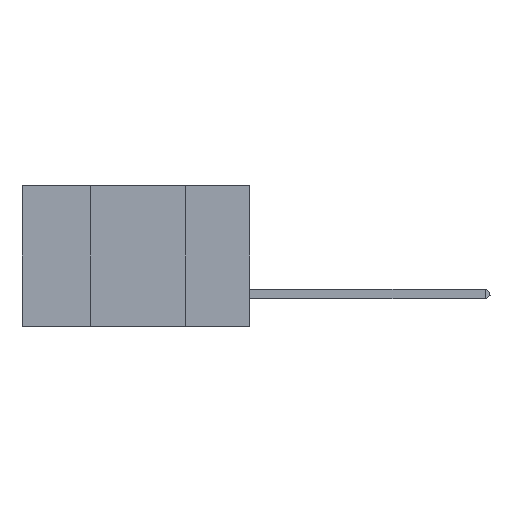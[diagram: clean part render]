
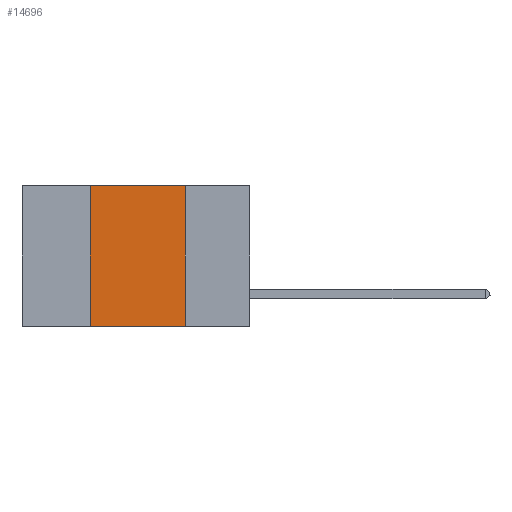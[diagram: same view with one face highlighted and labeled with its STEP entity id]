
A CAD part, left-side view. The second image highlights one B-rep face of the part: STEP entity #14696.
In plain terms, the highlighted planar face has unit normal (-1, 0, 0).
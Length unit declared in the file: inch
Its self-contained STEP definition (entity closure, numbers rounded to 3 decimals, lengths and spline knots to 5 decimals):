
#345 = LINE ( 'NONE', #9180, #18516 ) ;
#493 = VECTOR ( 'NONE', #5244, 39.37008 ) ;
#888 = VERTEX_POINT ( 'NONE', #1486 ) ;
#1486 = CARTESIAN_POINT ( 'NONE',  ( 0., 0.17, -0.37 ) ) ;
#1502 = CARTESIAN_POINT ( 'NONE',  ( 0., 0.6, -0.37 ) ) ;
#2614 = DIRECTION ( 'NONE',  ( 0., 0., 1. ) ) ;
#3941 = DIRECTION ( 'NONE',  ( 0., 0., -1. ) ) ;
#4021 = LINE ( 'NONE', #1502, #16399 ) ;
#4168 = DIRECTION ( 'NONE',  ( 1., 0., 0. ) ) ;
#4322 = VECTOR ( 'NONE', #19397, 39.37008 ) ;
#5244 = DIRECTION ( 'NONE',  ( 0., -1., 0. ) ) ;
#5332 = EDGE_CURVE ( 'NONE', #5375, #17509, #345, .T. ) ;
#5375 = VERTEX_POINT ( 'NONE', #17888 ) ;
#6744 = ORIENTED_EDGE ( 'NONE', *, *, #5332, .F. ) ;
#7427 = ORIENTED_EDGE ( 'NONE', *, *, #18509, .F. ) ;
#8189 = AXIS2_PLACEMENT_3D ( 'NONE', #19350, #4168, #3941 ) ;
#8877 = ORIENTED_EDGE ( 'NONE', *, *, #14952, .F. ) ;
#9180 = CARTESIAN_POINT ( 'NONE',  ( 0., 0.42, 0. ) ) ;
#10536 = LINE ( 'NONE', #15201, #493 ) ;
#12837 = EDGE_CURVE ( 'NONE', #5375, #888, #4021, .T. ) ;
#12891 = FACE_OUTER_BOUND ( 'NONE', #15866, .T. ) ;
#13281 = LINE ( 'NONE', #19268, #4322 ) ;
#14696 = ADVANCED_FACE ( 'NONE', ( #12891 ), #20930, .F. ) ;
#14952 = EDGE_CURVE ( 'NONE', #17509, #15002, #10536, .T. ) ;
#15002 = VERTEX_POINT ( 'NONE', #17249 ) ;
#15201 = CARTESIAN_POINT ( 'NONE',  ( 0., 0.6, 0. ) ) ;
#15866 = EDGE_LOOP ( 'NONE', ( #7427, #8877, #6744, #16803 ) ) ;
#16399 = VECTOR ( 'NONE', #19965, 39.37008 ) ;
#16803 = ORIENTED_EDGE ( 'NONE', *, *, #12837, .T. ) ;
#17249 = CARTESIAN_POINT ( 'NONE',  ( 0., 0.17, 0. ) ) ;
#17509 = VERTEX_POINT ( 'NONE', #17569 ) ;
#17569 = CARTESIAN_POINT ( 'NONE',  ( 0., 0.42, 0. ) ) ;
#17888 = CARTESIAN_POINT ( 'NONE',  ( 0., 0.42, -0.37 ) ) ;
#18509 = EDGE_CURVE ( 'NONE', #15002, #888, #13281, .T. ) ;
#18516 = VECTOR ( 'NONE', #2614, 39.37008 ) ;
#19268 = CARTESIAN_POINT ( 'NONE',  ( 0., 0.17, 0. ) ) ;
#19350 = CARTESIAN_POINT ( 'NONE',  ( 0., 0.6, 0. ) ) ;
#19397 = DIRECTION ( 'NONE',  ( 0., 0., -1. ) ) ;
#19965 = DIRECTION ( 'NONE',  ( 0., -1., 0. ) ) ;
#20930 = PLANE ( 'NONE',  #8189 ) ;
